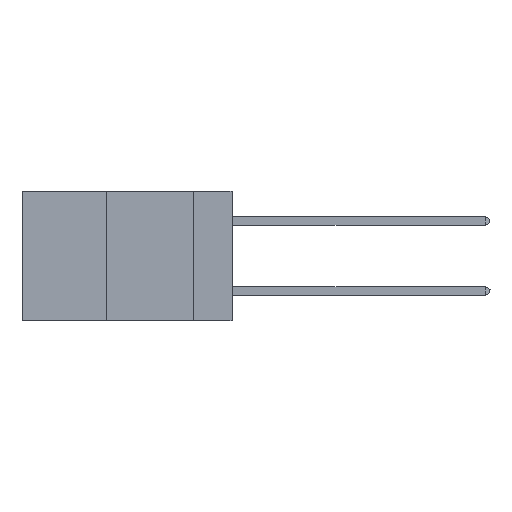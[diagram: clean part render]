
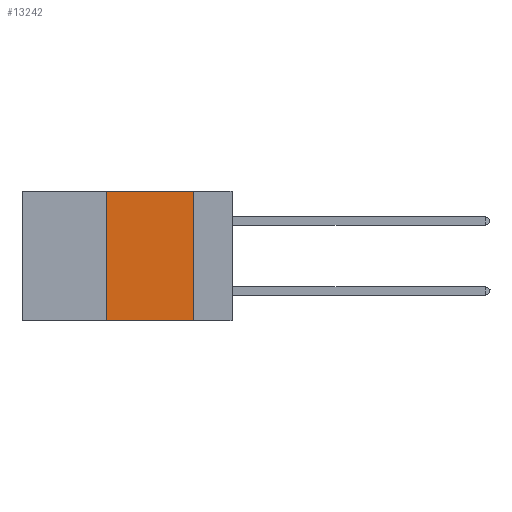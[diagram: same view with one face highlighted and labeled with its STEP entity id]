
A CAD part, left-side view. The second image highlights one B-rep face of the part: STEP entity #13242.
In plain terms, the highlighted planar face has unit normal (-1, 0, 0).
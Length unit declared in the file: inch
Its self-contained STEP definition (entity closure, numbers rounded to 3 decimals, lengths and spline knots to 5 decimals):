
#75 = VERTEX_POINT ( 'NONE', #960 ) ;
#283 = VERTEX_POINT ( 'NONE', #307 ) ;
#307 = CARTESIAN_POINT ( 'NONE',  ( 0., 0.36, -0.37 ) ) ;
#655 = ORIENTED_EDGE ( 'NONE', *, *, #6336, .T. ) ;
#697 = CARTESIAN_POINT ( 'NONE',  ( 0., 0.6, 0. ) ) ;
#960 = CARTESIAN_POINT ( 'NONE',  ( 0., 0.36, 0. ) ) ;
#1182 = FACE_OUTER_BOUND ( 'NONE', #5260, .T. ) ;
#1232 = CARTESIAN_POINT ( 'NONE',  ( 0., 0.11, 0. ) ) ;
#2370 = DIRECTION ( 'NONE',  ( 1., 0., 0. ) ) ;
#2450 = CARTESIAN_POINT ( 'NONE',  ( 0., 0.11, 0. ) ) ;
#2601 = CARTESIAN_POINT ( 'NONE',  ( 0., 0.6, -0.37 ) ) ;
#3329 = VERTEX_POINT ( 'NONE', #13791 ) ;
#3361 = CARTESIAN_POINT ( 'NONE',  ( 0., 0.36, 0. ) ) ;
#5260 = EDGE_LOOP ( 'NONE', ( #12155, #11371, #9311, #655 ) ) ;
#6336 = EDGE_CURVE ( 'NONE', #283, #3329, #13040, .T. ) ;
#6970 = AXIS2_PLACEMENT_3D ( 'NONE', #697, #2370, #13104 ) ;
#7193 = VECTOR ( 'NONE', #11042, 39.37008 ) ;
#8528 = LINE ( 'NONE', #10308, #15512 ) ;
#8633 = VECTOR ( 'NONE', #17797, 39.37008 ) ;
#9099 = EDGE_CURVE ( 'NONE', #75, #14150, #8528, .T. ) ;
#9311 = ORIENTED_EDGE ( 'NONE', *, *, #16024, .F. ) ;
#10308 = CARTESIAN_POINT ( 'NONE',  ( 0., 0.6, 0. ) ) ;
#10494 = EDGE_CURVE ( 'NONE', #14150, #3329, #19607, .T. ) ;
#11042 = DIRECTION ( 'NONE',  ( 0., 0., 1. ) ) ;
#11118 = LINE ( 'NONE', #3361, #7193 ) ;
#11371 = ORIENTED_EDGE ( 'NONE', *, *, #9099, .F. ) ;
#11733 = DIRECTION ( 'NONE',  ( 0., 0., -1. ) ) ;
#12155 = ORIENTED_EDGE ( 'NONE', *, *, #10494, .F. ) ;
#13040 = LINE ( 'NONE', #2601, #8633 ) ;
#13104 = DIRECTION ( 'NONE',  ( 0., 0., -1. ) ) ;
#13242 = ADVANCED_FACE ( 'NONE', ( #1182 ), #18986, .F. ) ;
#13791 = CARTESIAN_POINT ( 'NONE',  ( 0., 0.11, -0.37 ) ) ;
#14150 = VERTEX_POINT ( 'NONE', #1232 ) ;
#15245 = VECTOR ( 'NONE', #11733, 39.37008 ) ;
#15512 = VECTOR ( 'NONE', #16300, 39.37008 ) ;
#16024 = EDGE_CURVE ( 'NONE', #283, #75, #11118, .T. ) ;
#16300 = DIRECTION ( 'NONE',  ( 0., -1., 0. ) ) ;
#17797 = DIRECTION ( 'NONE',  ( 0., -1., 0. ) ) ;
#18986 = PLANE ( 'NONE',  #6970 ) ;
#19607 = LINE ( 'NONE', #2450, #15245 ) ;
